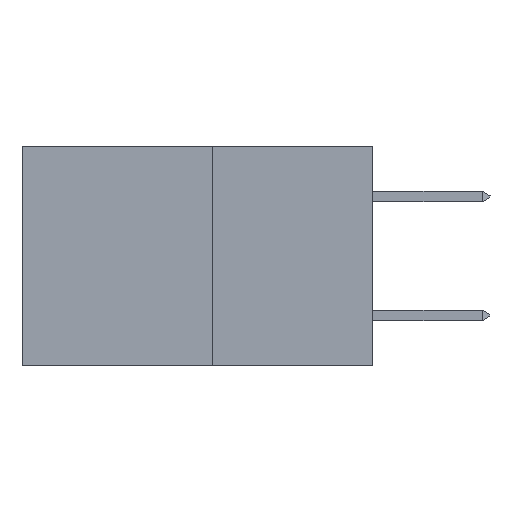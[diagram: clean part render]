
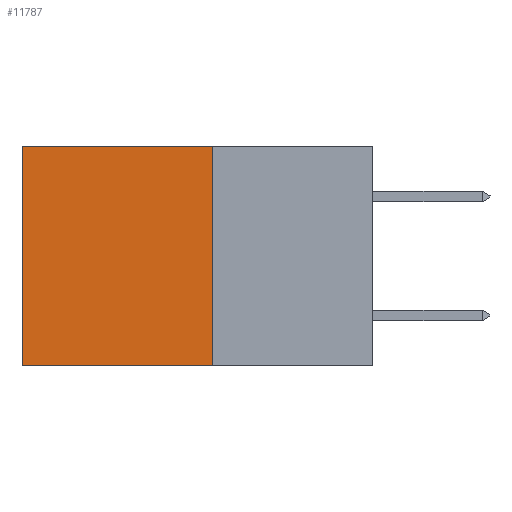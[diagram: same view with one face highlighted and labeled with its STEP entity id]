
A CAD part, left-side view. The second image highlights one B-rep face of the part: STEP entity #11787.
In plain terms, the highlighted planar face has unit normal (-1, 0, 0).
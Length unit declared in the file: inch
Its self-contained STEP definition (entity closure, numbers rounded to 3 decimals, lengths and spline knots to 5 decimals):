
#488 = DIRECTION ( 'NONE',  ( 0., 0., -1. ) ) ;
#1784 = EDGE_LOOP ( 'NONE', ( #13031, #16816, #5526, #1888 ) ) ;
#1888 = ORIENTED_EDGE ( 'NONE', *, *, #9578, .T. ) ;
#2210 = DIRECTION ( 'NONE',  ( 0., 0., -1. ) ) ;
#2363 = CARTESIAN_POINT ( 'NONE',  ( 0.277, 0.59, 0. ) ) ;
#2555 = VERTEX_POINT ( 'NONE', #10103 ) ;
#2608 = CARTESIAN_POINT ( 'NONE',  ( 0.277, 0.27, 0. ) ) ;
#3088 = CARTESIAN_POINT ( 'NONE',  ( 0.277, 0.27, -0.37 ) ) ;
#4010 = LINE ( 'NONE', #16590, #10802 ) ;
#4250 = CARTESIAN_POINT ( 'NONE',  ( 0.277, 0.27, -0.37 ) ) ;
#4973 = VECTOR ( 'NONE', #6959, 39.37008 ) ;
#5118 = EDGE_CURVE ( 'NONE', #12979, #6219, #14135, .T. ) ;
#5401 = LINE ( 'NONE', #5590, #4973 ) ;
#5526 = ORIENTED_EDGE ( 'NONE', *, *, #5118, .F. ) ;
#5590 = CARTESIAN_POINT ( 'NONE',  ( 0.277, 0.27, 0. ) ) ;
#6219 = VERTEX_POINT ( 'NONE', #14599 ) ;
#6886 = AXIS2_PLACEMENT_3D ( 'NONE', #9006, #10339, #2210 ) ;
#6959 = DIRECTION ( 'NONE',  ( 0., 1., 0. ) ) ;
#7398 = VERTEX_POINT ( 'NONE', #2363 ) ;
#8035 = FACE_OUTER_BOUND ( 'NONE', #1784, .T. ) ;
#8916 = LINE ( 'NONE', #4250, #15524 ) ;
#9006 = CARTESIAN_POINT ( 'NONE',  ( 0.277, 0.27, -0.37 ) ) ;
#9578 = EDGE_CURVE ( 'NONE', #12979, #7398, #5401, .T. ) ;
#10103 = CARTESIAN_POINT ( 'NONE',  ( 0.277, 0.59, -0.37 ) ) ;
#10113 = EDGE_CURVE ( 'NONE', #6219, #2555, #8916, .T. ) ;
#10339 = DIRECTION ( 'NONE',  ( 1., 0., 0. ) ) ;
#10802 = VECTOR ( 'NONE', #488, 39.37008 ) ;
#10894 = EDGE_CURVE ( 'NONE', #7398, #2555, #4010, .T. ) ;
#11062 = DIRECTION ( 'NONE',  ( 0., 1., 0. ) ) ;
#11221 = DIRECTION ( 'NONE',  ( 0., 0., -1. ) ) ;
#11787 = ADVANCED_FACE ( 'NONE', ( #8035 ), #16894, .F. ) ;
#12979 = VERTEX_POINT ( 'NONE', #2608 ) ;
#13031 = ORIENTED_EDGE ( 'NONE', *, *, #10894, .T. ) ;
#14135 = LINE ( 'NONE', #3088, #14545 ) ;
#14545 = VECTOR ( 'NONE', #11221, 39.37008 ) ;
#14599 = CARTESIAN_POINT ( 'NONE',  ( 0.277, 0.27, -0.37 ) ) ;
#15524 = VECTOR ( 'NONE', #11062, 39.37008 ) ;
#16590 = CARTESIAN_POINT ( 'NONE',  ( 0.277, 0.59, -0.37 ) ) ;
#16816 = ORIENTED_EDGE ( 'NONE', *, *, #10113, .F. ) ;
#16894 = PLANE ( 'NONE',  #6886 ) ;
